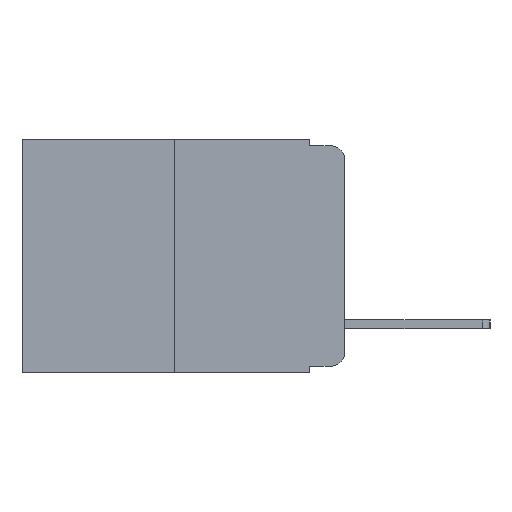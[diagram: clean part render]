
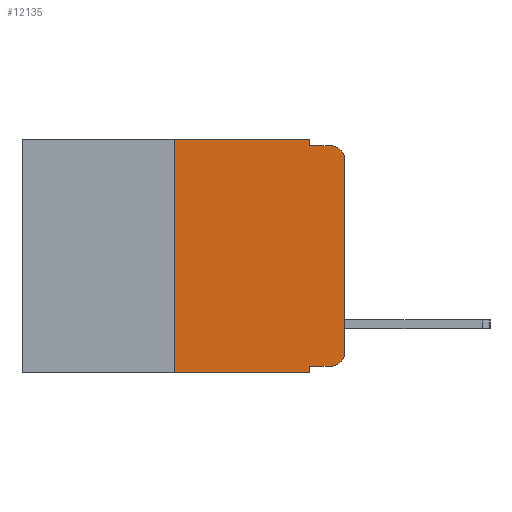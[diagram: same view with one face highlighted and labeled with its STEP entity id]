
A CAD part, left-side view. The second image highlights one B-rep face of the part: STEP entity #12135.
In plain terms, the highlighted planar face has unit normal (-1, 0, 0).
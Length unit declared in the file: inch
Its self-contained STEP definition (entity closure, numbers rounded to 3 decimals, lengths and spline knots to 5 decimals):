
#416 = CIRCLE ( 'NONE', #22183, 0.02 ) ;
#605 = LINE ( 'NONE', #15024, #20719 ) ;
#1064 = ORIENTED_EDGE ( 'NONE', *, *, #20051, .F. ) ;
#1331 = VECTOR ( 'NONE', #6199, 39.37008 ) ;
#1491 = VECTOR ( 'NONE', #12929, 39.37008 ) ;
#1502 = VECTOR ( 'NONE', #12649, 39.37008 ) ;
#1831 = CARTESIAN_POINT ( 'NONE',  ( 0., 0.473, 0. ) ) ;
#2043 = CARTESIAN_POINT ( 'NONE',  ( 0., 0.25, 0. ) ) ;
#2137 = LINE ( 'NONE', #2753, #1502 ) ;
#2665 = VECTOR ( 'NONE', #21248, 39.37008 ) ;
#2753 = CARTESIAN_POINT ( 'NONE',  ( 0., 0.051, 0. ) ) ;
#3019 = EDGE_CURVE ( 'NONE', #23848, #6619, #20978, .T. ) ;
#3340 = CARTESIAN_POINT ( 'NONE',  ( 0., 0., -0.313 ) ) ;
#3659 = CARTESIAN_POINT ( 'NONE',  ( 0., 0.051, -0.01 ) ) ;
#3849 = DIRECTION ( 'NONE',  ( 0., 0., -1. ) ) ;
#4809 = ORIENTED_EDGE ( 'NONE', *, *, #13765, .T. ) ;
#5006 = CARTESIAN_POINT ( 'NONE',  ( 0., 0.25, 0. ) ) ;
#5081 = CARTESIAN_POINT ( 'NONE',  ( 0., 0.051, 0. ) ) ;
#5338 = CARTESIAN_POINT ( 'NONE',  ( 0., 0.051, -0.343 ) ) ;
#5688 = ORIENTED_EDGE ( 'NONE', *, *, #16136, .F. ) ;
#5701 = CARTESIAN_POINT ( 'NONE',  ( 0., 0., 0. ) ) ;
#5746 = PLANE ( 'NONE',  #22656 ) ;
#6054 = LINE ( 'NONE', #18533, #15842 ) ;
#6199 = DIRECTION ( 'NONE',  ( 0., -1., 0. ) ) ;
#6273 = ORIENTED_EDGE ( 'NONE', *, *, #17421, .T. ) ;
#6619 = VERTEX_POINT ( 'NONE', #2043 ) ;
#6633 = LINE ( 'NONE', #14055, #1331 ) ;
#6694 = ORIENTED_EDGE ( 'NONE', *, *, #12461, .T. ) ;
#6870 = CARTESIAN_POINT ( 'NONE',  ( 0., 0.02, -0.313 ) ) ;
#7024 = EDGE_CURVE ( 'NONE', #15185, #14228, #2137, .T. ) ;
#7507 = VERTEX_POINT ( 'NONE', #23505 ) ;
#8500 = ORIENTED_EDGE ( 'NONE', *, *, #7024, .F. ) ;
#8616 = EDGE_LOOP ( 'NONE', ( #6273, #23178, #23489, #8500, #5688, #22909, #16699, #1064, #4809, #6694 ) ) ;
#8888 = DIRECTION ( 'NONE',  ( 0., 0., -1. ) ) ;
#9710 = EDGE_CURVE ( 'NONE', #14228, #18553, #13610, .T. ) ;
#9977 = CARTESIAN_POINT ( 'NONE',  ( 0., 0.02, -0.01 ) ) ;
#10214 = VERTEX_POINT ( 'NONE', #3340 ) ;
#11006 = EDGE_CURVE ( 'NONE', #7507, #18553, #14147, .T. ) ;
#11875 = DIRECTION ( 'NONE',  ( -1., 0., 0. ) ) ;
#12026 = CARTESIAN_POINT ( 'NONE',  ( 0., 0.25, -0.343 ) ) ;
#12135 = ADVANCED_FACE ( 'NONE', ( #22042 ), #5746, .F. ) ;
#12461 = EDGE_CURVE ( 'NONE', #21042, #10214, #416, .T. ) ;
#12649 = DIRECTION ( 'NONE',  ( 0., 0., -1. ) ) ;
#12810 = CARTESIAN_POINT ( 'NONE',  ( 0., 0.02, -0.333 ) ) ;
#12929 = DIRECTION ( 'NONE',  ( 0., 0., 1. ) ) ;
#13610 = LINE ( 'NONE', #20894, #23083 ) ;
#13765 = EDGE_CURVE ( 'NONE', #17487, #21042, #6633, .T. ) ;
#14055 = CARTESIAN_POINT ( 'NONE',  ( 0., 0.051, -0.333 ) ) ;
#14147 = CIRCLE ( 'NONE', #19422, 0.02 ) ;
#14228 = VERTEX_POINT ( 'NONE', #3659 ) ;
#15024 = CARTESIAN_POINT ( 'NONE',  ( 0., 0.051, 0. ) ) ;
#15185 = VERTEX_POINT ( 'NONE', #5081 ) ;
#15280 = VERTEX_POINT ( 'NONE', #5338 ) ;
#15397 = DIRECTION ( 'NONE',  ( 0., -1., 0. ) ) ;
#15607 = DIRECTION ( 'NONE',  ( 1., 0., 0. ) ) ;
#15842 = VECTOR ( 'NONE', #20425, 39.37008 ) ;
#16136 = EDGE_CURVE ( 'NONE', #6619, #15185, #24206, .T. ) ;
#16699 = ORIENTED_EDGE ( 'NONE', *, *, #22193, .T. ) ;
#16883 = DIRECTION ( 'NONE',  ( 0., 0., -1. ) ) ;
#17421 = EDGE_CURVE ( 'NONE', #10214, #7507, #23295, .T. ) ;
#17487 = VERTEX_POINT ( 'NONE', #21323 ) ;
#18533 = CARTESIAN_POINT ( 'NONE',  ( 0., 0.473, -0.343 ) ) ;
#18553 = VERTEX_POINT ( 'NONE', #9977 ) ;
#19422 = AXIS2_PLACEMENT_3D ( 'NONE', #23268, #11875, #25134 ) ;
#20051 = EDGE_CURVE ( 'NONE', #17487, #15280, #605, .T. ) ;
#20338 = DIRECTION ( 'NONE',  ( -1., 0., 0. ) ) ;
#20425 = DIRECTION ( 'NONE',  ( 0., -1., 0. ) ) ;
#20719 = VECTOR ( 'NONE', #16883, 39.37008 ) ;
#20894 = CARTESIAN_POINT ( 'NONE',  ( 0., 0.051, -0.01 ) ) ;
#20901 = CARTESIAN_POINT ( 'NONE',  ( 0., 0.473, 0. ) ) ;
#20978 = LINE ( 'NONE', #5006, #1491 ) ;
#21042 = VERTEX_POINT ( 'NONE', #12810 ) ;
#21248 = DIRECTION ( 'NONE',  ( 0., 0., 1. ) ) ;
#21323 = CARTESIAN_POINT ( 'NONE',  ( 0., 0.051, -0.333 ) ) ;
#22042 = FACE_OUTER_BOUND ( 'NONE', #8616, .T. ) ;
#22183 = AXIS2_PLACEMENT_3D ( 'NONE', #6870, #20338, #8888 ) ;
#22193 = EDGE_CURVE ( 'NONE', #23848, #15280, #6054, .T. ) ;
#22656 = AXIS2_PLACEMENT_3D ( 'NONE', #1831, #15607, #3849 ) ;
#22796 = DIRECTION ( 'NONE',  ( 0., -1., 0. ) ) ;
#22909 = ORIENTED_EDGE ( 'NONE', *, *, #3019, .F. ) ;
#23025 = VECTOR ( 'NONE', #15397, 39.37008 ) ;
#23083 = VECTOR ( 'NONE', #22796, 39.37008 ) ;
#23178 = ORIENTED_EDGE ( 'NONE', *, *, #11006, .T. ) ;
#23268 = CARTESIAN_POINT ( 'NONE',  ( 0., 0.02, -0.03 ) ) ;
#23295 = LINE ( 'NONE', #5701, #2665 ) ;
#23489 = ORIENTED_EDGE ( 'NONE', *, *, #9710, .F. ) ;
#23505 = CARTESIAN_POINT ( 'NONE',  ( 0., 0., -0.03 ) ) ;
#23848 = VERTEX_POINT ( 'NONE', #12026 ) ;
#24206 = LINE ( 'NONE', #20901, #23025 ) ;
#25134 = DIRECTION ( 'NONE',  ( 0., 0., -1. ) ) ;
